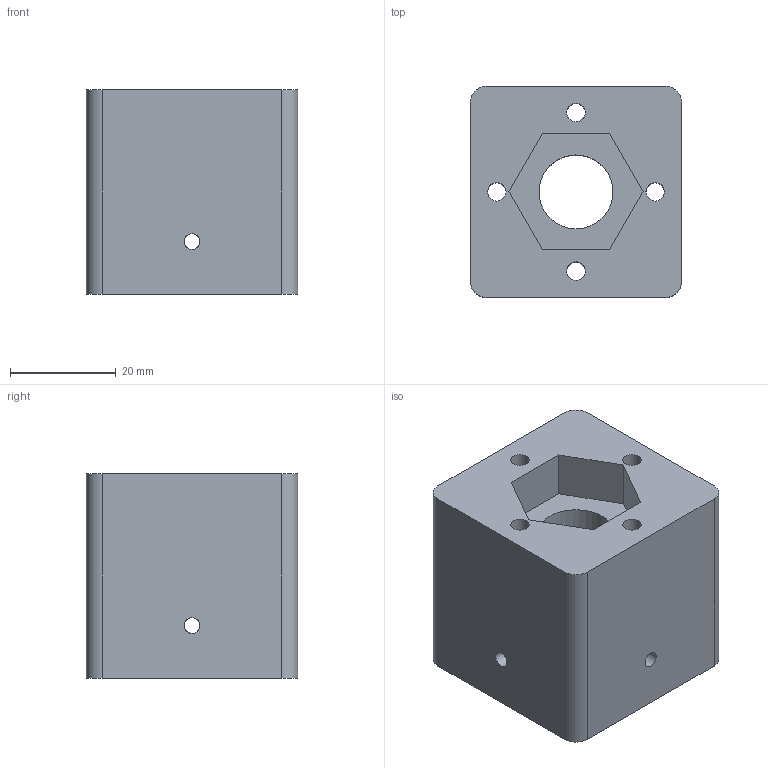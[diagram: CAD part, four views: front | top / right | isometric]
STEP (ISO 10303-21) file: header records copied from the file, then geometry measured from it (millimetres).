
FILE_DESCRIPTION(/* description */ (''),/* implementation_level */ '2;1');
FILE_NAME(/* name */ 'M14 Bolt Jig STEP.step',/* time_stamp */ '2022-08-27T22:40:39-04:00',/* author */ (''),/* organization */ (''),/* preprocessor_version */ 'ST-DEVELOPER v19',/* originating_system */ 'Autodesk Translation Framework v11.7.0.108',/* authorisation */ '');
FILE_SCHEMA (('AUTOMOTIVE_DESIGN { 1 0 10303 214 3 1 1 }'));
Length unit declared in the file: millimetre
Products named in the file (1): HiLo JIG_M14 Bolt Jig
Bounding box: 40 x 40 x 38.8 mm (x, y, z)
Volume: 51647.3 mm3; surface area: 12780.6 mm2
Topology: 1 solids, 1 shells, 30 faces, 94 edges, 64 vertices
Faces by surface type: cylinder 17, plane 13
Full cylindrical faces by diameter (mm): 3 x8, 3.5 x4, 14 x1
Entity records: 1563 total; most frequent: CARTESIAN_POINT 659, ORIENTED_EDGE 188, DIRECTION 156, EDGE_CURVE 94, VERTEX_POINT 64, EDGE_LOOP 54, AXIS2_PLACEMENT_3D 53, LINE 50
